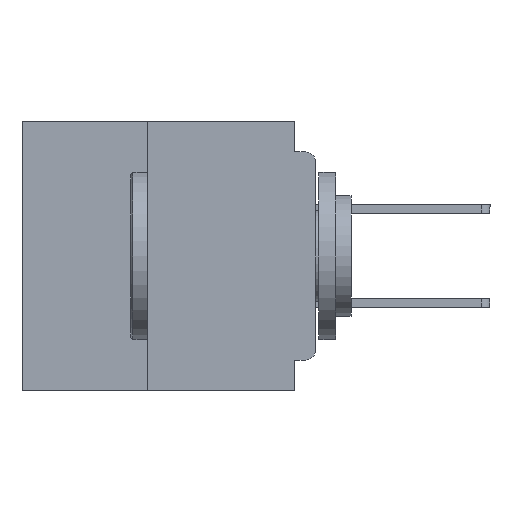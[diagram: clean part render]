
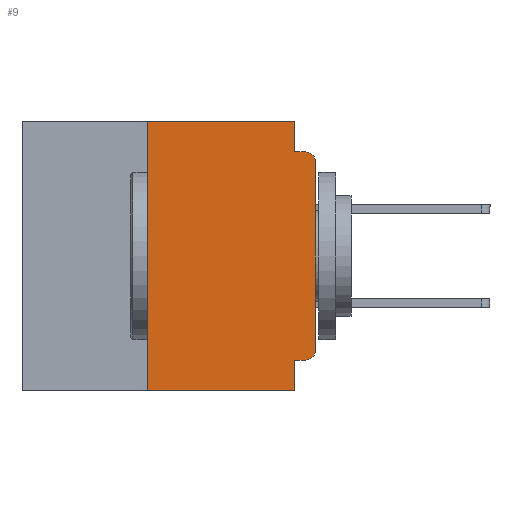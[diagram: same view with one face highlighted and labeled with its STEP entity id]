
A CAD part, left-side view. The second image highlights one B-rep face of the part: STEP entity #9.
In plain terms, the highlighted planar face has unit normal (-1, 0, 0).
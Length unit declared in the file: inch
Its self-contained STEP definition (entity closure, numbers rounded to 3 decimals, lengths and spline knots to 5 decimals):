
#9 = ADVANCED_FACE ( 'NONE', ( #16165 ), #25781, .F. ) ;
#286 = EDGE_CURVE ( 'NONE', #37018, #325, #33107, .T. ) ;
#325 = VERTEX_POINT ( 'NONE', #20215 ) ;
#1772 = CARTESIAN_POINT ( 'NONE',  ( 0., 0.437, -0.4 ) ) ;
#2018 = DIRECTION ( 'NONE',  ( 0., -1., 0. ) ) ;
#2287 = CARTESIAN_POINT ( 'NONE',  ( 0., 0.015, -0.355 ) ) ;
#3080 = CARTESIAN_POINT ( 'NONE',  ( 0., 0., -0.045 ) ) ;
#3219 = LINE ( 'NONE', #16314, #39484 ) ;
#4308 = EDGE_CURVE ( 'NONE', #10539, #34720, #43630, .T. ) ;
#5415 = ORIENTED_EDGE ( 'NONE', *, *, #25573, .F. ) ;
#5673 = DIRECTION ( 'NONE',  ( 0., 0., 1. ) ) ;
#8506 = ORIENTED_EDGE ( 'NONE', *, *, #286, .T. ) ;
#8751 = ORIENTED_EDGE ( 'NONE', *, *, #36005, .F. ) ;
#9462 = VECTOR ( 'NONE', #37046, 39.37008 ) ;
#9860 = CARTESIAN_POINT ( 'NONE',  ( 0., 0., 0. ) ) ;
#10065 = DIRECTION ( 'NONE',  ( -1., 0., 0. ) ) ;
#10224 = CIRCLE ( 'NONE', #29916, 0.015 ) ;
#10539 = VERTEX_POINT ( 'NONE', #39574 ) ;
#10563 = LINE ( 'NONE', #19619, #9462 ) ;
#11330 = DIRECTION ( 'NONE',  ( -1., 0., 0. ) ) ;
#12101 = ORIENTED_EDGE ( 'NONE', *, *, #23619, .F. ) ;
#12112 = VERTEX_POINT ( 'NONE', #38229 ) ;
#13415 = CARTESIAN_POINT ( 'NONE',  ( 0., 0.031, -0.4 ) ) ;
#14303 = ORIENTED_EDGE ( 'NONE', *, *, #25204, .F. ) ;
#14345 = LINE ( 'NONE', #15403, #34060 ) ;
#15121 = VERTEX_POINT ( 'NONE', #2287 ) ;
#15403 = CARTESIAN_POINT ( 'NONE',  ( 0., 0., -0.355 ) ) ;
#16165 = FACE_OUTER_BOUND ( 'NONE', #25943, .T. ) ;
#16314 = CARTESIAN_POINT ( 'NONE',  ( 0., 0.437, 0. ) ) ;
#16448 = VECTOR ( 'NONE', #25649, 39.37008 ) ;
#17601 = LINE ( 'NONE', #3080, #44323 ) ;
#18151 = ORIENTED_EDGE ( 'NONE', *, *, #20323, .F. ) ;
#19619 = CARTESIAN_POINT ( 'NONE',  ( 0., 0.25, -0.4 ) ) ;
#19830 = DIRECTION ( 'NONE',  ( 0., -1., 0. ) ) ;
#20215 = CARTESIAN_POINT ( 'NONE',  ( 0., 0., -0.06 ) ) ;
#20323 = EDGE_CURVE ( 'NONE', #10539, #36521, #10563, .T. ) ;
#20438 = AXIS2_PLACEMENT_3D ( 'NONE', #32347, #11330, #35804 ) ;
#22079 = CARTESIAN_POINT ( 'NONE',  ( 0., 0.031, 0. ) ) ;
#23619 = EDGE_CURVE ( 'NONE', #12112, #34720, #27695, .T. ) ;
#25122 = VERTEX_POINT ( 'NONE', #42687 ) ;
#25178 = VECTOR ( 'NONE', #2018, 39.37008 ) ;
#25204 = EDGE_CURVE ( 'NONE', #15121, #12112, #14345, .T. ) ;
#25573 = EDGE_CURVE ( 'NONE', #33007, #25122, #17601, .T. ) ;
#25649 = DIRECTION ( 'NONE',  ( 0., 0., -1. ) ) ;
#25781 = PLANE ( 'NONE',  #35068 ) ;
#25943 = EDGE_LOOP ( 'NONE', ( #8506, #27264, #5415, #35615, #8751, #18151, #38909, #12101, #14303, #32947 ) ) ;
#26191 = DIRECTION ( 'NONE',  ( 1., 0., 0. ) ) ;
#26286 = CARTESIAN_POINT ( 'NONE',  ( 0., 0.437, 0. ) ) ;
#26388 = DIRECTION ( 'NONE',  ( 0., 0., -1. ) ) ;
#26638 = VECTOR ( 'NONE', #27604, 39.37008 ) ;
#27264 = ORIENTED_EDGE ( 'NONE', *, *, #35595, .T. ) ;
#27604 = DIRECTION ( 'NONE',  ( 0., 0., -1. ) ) ;
#27695 = LINE ( 'NONE', #34432, #26638 ) ;
#27772 = DIRECTION ( 'NONE',  ( 0., -1., 0. ) ) ;
#28302 = EDGE_CURVE ( 'NONE', #15121, #37018, #10224, .T. ) ;
#28596 = CIRCLE ( 'NONE', #20438, 0.015 ) ;
#29916 = AXIS2_PLACEMENT_3D ( 'NONE', #31095, #10065, #34587 ) ;
#31095 = CARTESIAN_POINT ( 'NONE',  ( 0., 0.015, -0.34 ) ) ;
#32022 = VECTOR ( 'NONE', #5673, 39.37008 ) ;
#32347 = CARTESIAN_POINT ( 'NONE',  ( 0., 0.015, -0.06 ) ) ;
#32947 = ORIENTED_EDGE ( 'NONE', *, *, #28302, .T. ) ;
#33007 = VERTEX_POINT ( 'NONE', #34940 ) ;
#33107 = LINE ( 'NONE', #9860, #32022 ) ;
#34060 = VECTOR ( 'NONE', #36318, 39.37008 ) ;
#34432 = CARTESIAN_POINT ( 'NONE',  ( 0., 0.031, -0.4 ) ) ;
#34587 = DIRECTION ( 'NONE',  ( 0., 0., -1. ) ) ;
#34720 = VERTEX_POINT ( 'NONE', #13415 ) ;
#34940 = CARTESIAN_POINT ( 'NONE',  ( 0., 0.031, -0.045 ) ) ;
#35068 = AXIS2_PLACEMENT_3D ( 'NONE', #26286, #26191, #26388 ) ;
#35595 = EDGE_CURVE ( 'NONE', #325, #25122, #28596, .T. ) ;
#35615 = ORIENTED_EDGE ( 'NONE', *, *, #36998, .F. ) ;
#35804 = DIRECTION ( 'NONE',  ( 0., 0., -1. ) ) ;
#36005 = EDGE_CURVE ( 'NONE', #36521, #43289, #3219, .T. ) ;
#36318 = DIRECTION ( 'NONE',  ( 0., 1., 0. ) ) ;
#36521 = VERTEX_POINT ( 'NONE', #43871 ) ;
#36998 = EDGE_CURVE ( 'NONE', #43289, #33007, #44260, .T. ) ;
#37018 = VERTEX_POINT ( 'NONE', #43067 ) ;
#37046 = DIRECTION ( 'NONE',  ( 0., 0., 1. ) ) ;
#38229 = CARTESIAN_POINT ( 'NONE',  ( 0., 0.031, -0.355 ) ) ;
#38909 = ORIENTED_EDGE ( 'NONE', *, *, #4308, .T. ) ;
#39484 = VECTOR ( 'NONE', #19830, 39.37008 ) ;
#39574 = CARTESIAN_POINT ( 'NONE',  ( 0., 0.25, -0.4 ) ) ;
#41680 = CARTESIAN_POINT ( 'NONE',  ( 0., 0.031, 0. ) ) ;
#42687 = CARTESIAN_POINT ( 'NONE',  ( 0., 0.015, -0.045 ) ) ;
#43067 = CARTESIAN_POINT ( 'NONE',  ( 0., 0., -0.34 ) ) ;
#43289 = VERTEX_POINT ( 'NONE', #41680 ) ;
#43630 = LINE ( 'NONE', #1772, #25178 ) ;
#43871 = CARTESIAN_POINT ( 'NONE',  ( 0., 0.25, 0. ) ) ;
#44260 = LINE ( 'NONE', #22079, #16448 ) ;
#44323 = VECTOR ( 'NONE', #27772, 39.37008 ) ;
